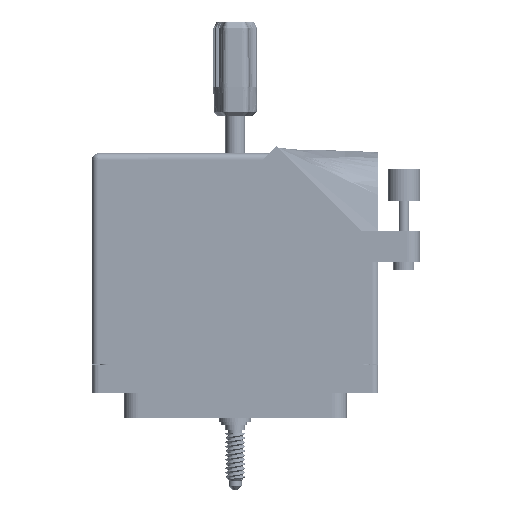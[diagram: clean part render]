
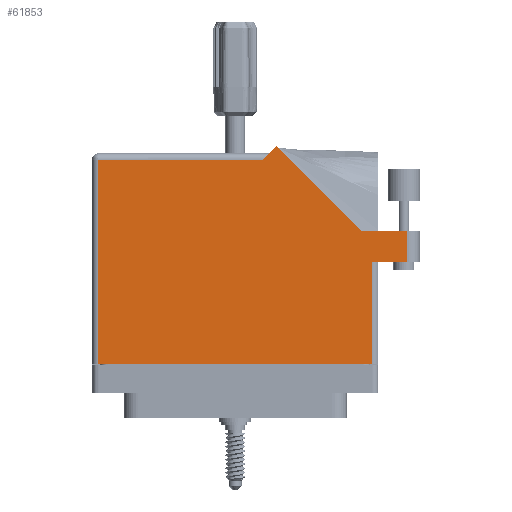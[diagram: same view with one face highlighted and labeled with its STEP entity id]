
A CAD part, front view. The second image highlights one B-rep face of the part: STEP entity #61853.
In plain terms, the highlighted face is planar.
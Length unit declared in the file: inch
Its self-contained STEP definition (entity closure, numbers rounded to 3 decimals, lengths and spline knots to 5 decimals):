
#2664 = CARTESIAN_POINT ( 'NONE',  ( -1.3155, -0.1, 0.765 ) ) ;
#3160 = EDGE_CURVE ( 'NONE', #28040, #11717, #70595, .T. ) ;
#3580 = ORIENTED_EDGE ( 'NONE', *, *, #84470, .T. ) ;
#3673 = FACE_OUTER_BOUND ( 'NONE', #32147, .T. ) ;
#4997 = VERTEX_POINT ( 'NONE', #21200 ) ;
#5604 = DIRECTION ( 'NONE',  ( -1., 0., 0. ) ) ;
#7289 = CARTESIAN_POINT ( 'NONE',  ( 1.6525, 1.187, 0.765 ) ) ;
#9127 = VERTEX_POINT ( 'NONE', #102928 ) ;
#9606 = EDGE_CURVE ( 'NONE', #59899, #87958, #88183, .T. ) ;
#9729 = VECTOR ( 'NONE', #5604, 39.37008 ) ;
#10850 = EDGE_CURVE ( 'NONE', #34408, #9127, #24647, .T. ) ;
#11717 = VERTEX_POINT ( 'NONE', #34531 ) ;
#12048 = LINE ( 'NONE', #77403, #9729 ) ;
#14076 = DIRECTION ( 'NONE',  ( -1., 0., 0. ) ) ;
#19357 = VECTOR ( 'NONE', #38386, 39.37008 ) ;
#21200 = CARTESIAN_POINT ( 'NONE',  ( 1.21192, 1.187, 0.765 ) ) ;
#22092 = LINE ( 'NONE', #87443, #77354 ) ;
#22381 = CARTESIAN_POINT ( 'NONE',  ( 1.3155, -0.1, 0.765 ) ) ;
#24647 = LINE ( 'NONE', #2664, #37333 ) ;
#25132 = VECTOR ( 'NONE', #88435, 39.37008 ) ;
#28040 = VERTEX_POINT ( 'NONE', #89579 ) ;
#30113 = LINE ( 'NONE', #61688, #34310 ) ;
#30712 = ORIENTED_EDGE ( 'NONE', *, *, #9606, .T. ) ;
#31448 = CARTESIAN_POINT ( 'NONE',  ( 0.3275, 1.93, 0.765 ) ) ;
#32147 = EDGE_LOOP ( 'NONE', ( #89803, #30712, #3580, #95372, #63688, #79245, #67133, #64502, #67062 ) ) ;
#33328 = LINE ( 'NONE', #97088, #79397 ) ;
#34310 = VECTOR ( 'NONE', #37578, 39.37008 ) ;
#34408 = VERTEX_POINT ( 'NONE', #48051 ) ;
#34531 = CARTESIAN_POINT ( 'NONE',  ( 0.2655, 1.868, 0.765 ) ) ;
#35321 = CARTESIAN_POINT ( 'NONE',  ( 1.6525, 0.88, 0.765 ) ) ;
#35969 = CARTESIAN_POINT ( 'NONE',  ( 1.3155, 0.88, 0.765 ) ) ;
#37333 = VECTOR ( 'NONE', #61008, 39.37008 ) ;
#37578 = DIRECTION ( 'NONE',  ( 0., 1., 0. ) ) ;
#37925 = VECTOR ( 'NONE', #85503, 39.37008 ) ;
#38386 = DIRECTION ( 'NONE',  ( 0., 1., 0. ) ) ;
#44342 = VERTEX_POINT ( 'NONE', #22381 ) ;
#44488 = VECTOR ( 'NONE', #102715, 39.37008 ) ;
#44603 = CARTESIAN_POINT ( 'NONE',  ( 1.6525, 1.187, 0.765 ) ) ;
#48051 = CARTESIAN_POINT ( 'NONE',  ( -1.3155, 1.868, 0.765 ) ) ;
#50613 = VERTEX_POINT ( 'NONE', #35969 ) ;
#56340 = DIRECTION ( 'NONE',  ( 1., 0., 0. ) ) ;
#58850 = DIRECTION ( 'NONE',  ( 0., 0., -1. ) ) ;
#59285 = LINE ( 'NONE', #100553, #37925 ) ;
#59388 = EDGE_CURVE ( 'NONE', #50613, #59899, #33328, .T. ) ;
#59899 = VERTEX_POINT ( 'NONE', #35321 ) ;
#61008 = DIRECTION ( 'NONE',  ( 0., -1., 0. ) ) ;
#61688 = CARTESIAN_POINT ( 'NONE',  ( 1.3155, 0.88, 0.765 ) ) ;
#61853 = ADVANCED_FACE ( 'NONE', ( #3673 ), #91524, .F. ) ;
#63688 = ORIENTED_EDGE ( 'NONE', *, *, #3160, .T. ) ;
#64502 = ORIENTED_EDGE ( 'NONE', *, *, #76917, .T. ) ;
#64665 = EDGE_CURVE ( 'NONE', #4997, #28040, #59285, .T. ) ;
#67062 = ORIENTED_EDGE ( 'NONE', *, *, #96917, .T. ) ;
#67133 = ORIENTED_EDGE ( 'NONE', *, *, #10850, .T. ) ;
#67423 = DIRECTION ( 'NONE',  ( -1., 0., 0. ) ) ;
#67605 = AXIS2_PLACEMENT_3D ( 'NONE', #100650, #58850, #67423 ) ;
#70595 = LINE ( 'NONE', #31448, #44488 ) ;
#76917 = EDGE_CURVE ( 'NONE', #9127, #44342, #97005, .T. ) ;
#77354 = VECTOR ( 'NONE', #14076, 39.37008 ) ;
#77403 = CARTESIAN_POINT ( 'NONE',  ( -1.3775, 1.868, 0.765 ) ) ;
#79245 = ORIENTED_EDGE ( 'NONE', *, *, #90822, .T. ) ;
#79397 = VECTOR ( 'NONE', #56340, 39.37008 ) ;
#84470 = EDGE_CURVE ( 'NONE', #87958, #4997, #22092, .T. ) ;
#85503 = DIRECTION ( 'NONE',  ( -0.707, 0.707, 0. ) ) ;
#87443 = CARTESIAN_POINT ( 'NONE',  ( 1.7775, 1.187, 0.765 ) ) ;
#87958 = VERTEX_POINT ( 'NONE', #44603 ) ;
#88183 = LINE ( 'NONE', #7289, #19357 ) ;
#88435 = DIRECTION ( 'NONE',  ( 1., 0., 0. ) ) ;
#89497 = CARTESIAN_POINT ( 'NONE',  ( -1.3775, -0.1, 0.765 ) ) ;
#89579 = CARTESIAN_POINT ( 'NONE',  ( 0.39821, 2.00071, 0.765 ) ) ;
#89803 = ORIENTED_EDGE ( 'NONE', *, *, #59388, .T. ) ;
#90822 = EDGE_CURVE ( 'NONE', #11717, #34408, #12048, .T. ) ;
#91524 = PLANE ( 'NONE',  #67605 ) ;
#95372 = ORIENTED_EDGE ( 'NONE', *, *, #64665, .T. ) ;
#96917 = EDGE_CURVE ( 'NONE', #44342, #50613, #30113, .T. ) ;
#97005 = LINE ( 'NONE', #89497, #25132 ) ;
#97088 = CARTESIAN_POINT ( 'NONE',  ( 1.3775, 0.88, 0.765 ) ) ;
#100553 = CARTESIAN_POINT ( 'NONE',  ( 1.21192, 1.187, 0.765 ) ) ;
#100650 = CARTESIAN_POINT ( 'NONE',  ( -1.3775, 1.93, 0.765 ) ) ;
#102715 = DIRECTION ( 'NONE',  ( -0.707, -0.707, 0. ) ) ;
#102928 = CARTESIAN_POINT ( 'NONE',  ( -1.3155, -0.1, 0.765 ) ) ;
